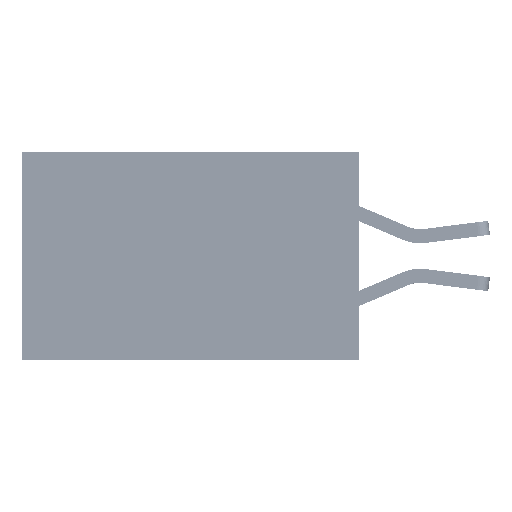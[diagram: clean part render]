
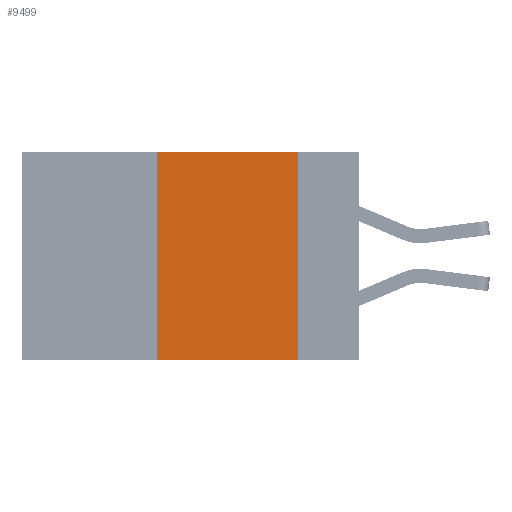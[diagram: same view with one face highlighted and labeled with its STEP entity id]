
A CAD part, left-side view. The second image highlights one B-rep face of the part: STEP entity #9499.
In plain terms, the highlighted planar face has unit normal (-1, 0, 0).
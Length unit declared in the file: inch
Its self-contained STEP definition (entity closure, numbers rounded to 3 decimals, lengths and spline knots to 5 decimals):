
#887 = DIRECTION ( 'NONE',  ( 0., 0., -1. ) ) ;
#2378 = VERTEX_POINT ( 'NONE', #21831 ) ;
#2447 = PLANE ( 'NONE',  #26256 ) ;
#2929 = ORIENTED_EDGE ( 'NONE', *, *, #26174, .F. ) ;
#4450 = ORIENTED_EDGE ( 'NONE', *, *, #10369, .F. ) ;
#4578 = VERTEX_POINT ( 'NONE', #27476 ) ;
#5607 = CARTESIAN_POINT ( 'NONE',  ( 0., 0.36, -0.37 ) ) ;
#5615 = DIRECTION ( 'NONE',  ( 0., -1., 0. ) ) ;
#6095 = DIRECTION ( 'NONE',  ( 1., 0., 0. ) ) ;
#6395 = CARTESIAN_POINT ( 'NONE',  ( 0., 0.36, 0. ) ) ;
#7397 = CARTESIAN_POINT ( 'NONE',  ( 0., 0.6, -0.37 ) ) ;
#8591 = LINE ( 'NONE', #7397, #36939 ) ;
#8953 = DIRECTION ( 'NONE',  ( 0., 0., -1. ) ) ;
#9499 = ADVANCED_FACE ( 'NONE', ( #10307 ), #2447, .F. ) ;
#10307 = FACE_OUTER_BOUND ( 'NONE', #16229, .T. ) ;
#10369 = EDGE_CURVE ( 'NONE', #2378, #4578, #20968, .T. ) ;
#13635 = VERTEX_POINT ( 'NONE', #6395 ) ;
#14342 = VECTOR ( 'NONE', #887, 39.37008 ) ;
#14804 = VERTEX_POINT ( 'NONE', #5607 ) ;
#15144 = LINE ( 'NONE', #18361, #34903 ) ;
#16229 = EDGE_LOOP ( 'NONE', ( #4450, #2929, #37854, #30421 ) ) ;
#16620 = DIRECTION ( 'NONE',  ( 0., 0., 1. ) ) ;
#17752 = DIRECTION ( 'NONE',  ( 0., -1., 0. ) ) ;
#18317 = LINE ( 'NONE', #39521, #39588 ) ;
#18361 = CARTESIAN_POINT ( 'NONE',  ( 0., 0.6, 0. ) ) ;
#20968 = LINE ( 'NONE', #33841, #14342 ) ;
#21831 = CARTESIAN_POINT ( 'NONE',  ( 0., 0.11, 0. ) ) ;
#25616 = EDGE_CURVE ( 'NONE', #14804, #4578, #8591, .T. ) ;
#26174 = EDGE_CURVE ( 'NONE', #13635, #2378, #15144, .T. ) ;
#26256 = AXIS2_PLACEMENT_3D ( 'NONE', #41207, #6095, #8953 ) ;
#27476 = CARTESIAN_POINT ( 'NONE',  ( 0., 0.11, -0.37 ) ) ;
#30421 = ORIENTED_EDGE ( 'NONE', *, *, #25616, .T. ) ;
#33841 = CARTESIAN_POINT ( 'NONE',  ( 0., 0.11, 0. ) ) ;
#34903 = VECTOR ( 'NONE', #5615, 39.37008 ) ;
#36939 = VECTOR ( 'NONE', #17752, 39.37008 ) ;
#37854 = ORIENTED_EDGE ( 'NONE', *, *, #41243, .F. ) ;
#39521 = CARTESIAN_POINT ( 'NONE',  ( 0., 0.36, 0. ) ) ;
#39588 = VECTOR ( 'NONE', #16620, 39.37008 ) ;
#41207 = CARTESIAN_POINT ( 'NONE',  ( 0., 0.6, 0. ) ) ;
#41243 = EDGE_CURVE ( 'NONE', #14804, #13635, #18317, .T. ) ;
